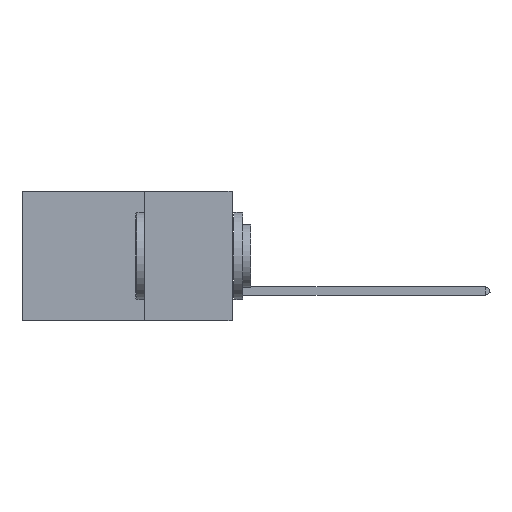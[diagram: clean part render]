
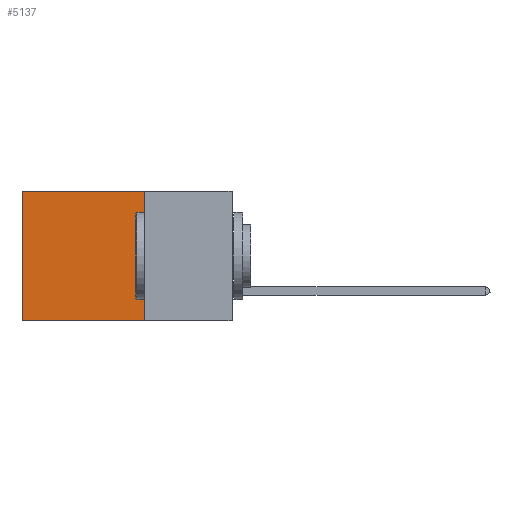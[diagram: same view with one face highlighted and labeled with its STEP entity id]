
A CAD part, left-side view. The second image highlights one B-rep face of the part: STEP entity #5137.
In plain terms, the highlighted planar face has unit normal (-1, 0, 0).
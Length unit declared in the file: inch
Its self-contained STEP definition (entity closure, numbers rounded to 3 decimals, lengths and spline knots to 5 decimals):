
#552 = LINE ( 'NONE', #20844, #25402 ) ;
#698 = CARTESIAN_POINT ( 'NONE',  ( 0.2875, 0.25, -0.37 ) ) ;
#1179 = DIRECTION ( 'NONE',  ( 0., 1., 0. ) ) ;
#1257 = LINE ( 'NONE', #7891, #14484 ) ;
#1474 = ORIENTED_EDGE ( 'NONE', *, *, #8886, .F. ) ;
#1738 = ORIENTED_EDGE ( 'NONE', *, *, #21145, .T. ) ;
#3791 = DIRECTION ( 'NONE',  ( 0., 0., -1. ) ) ;
#5137 = ADVANCED_FACE ( 'NONE', ( #21588 ), #13973, .F. ) ;
#6836 = EDGE_CURVE ( 'NONE', #13705, #20027, #1257, .T. ) ;
#7587 = CARTESIAN_POINT ( 'NONE',  ( 0.2875, 0.6, 0. ) ) ;
#7891 = CARTESIAN_POINT ( 'NONE',  ( 0.2875, 0.25, 0. ) ) ;
#8006 = CARTESIAN_POINT ( 'NONE',  ( 0.2875, 0.6, -0.37 ) ) ;
#8116 = VERTEX_POINT ( 'NONE', #698 ) ;
#8886 = EDGE_CURVE ( 'NONE', #8116, #20787, #552, .T. ) ;
#9477 = VECTOR ( 'NONE', #13708, 39.37008 ) ;
#11880 = DIRECTION ( 'NONE',  ( 0., 1., 0. ) ) ;
#13496 = CARTESIAN_POINT ( 'NONE',  ( 0.2875, 0.25, 0. ) ) ;
#13705 = VERTEX_POINT ( 'NONE', #17081 ) ;
#13708 = DIRECTION ( 'NONE',  ( 0., 0., -1. ) ) ;
#13969 = AXIS2_PLACEMENT_3D ( 'NONE', #22294, #14064, #3791 ) ;
#13973 = PLANE ( 'NONE',  #13969 ) ;
#14064 = DIRECTION ( 'NONE',  ( 1., 0., 0. ) ) ;
#14484 = VECTOR ( 'NONE', #11880, 39.37008 ) ;
#14541 = CARTESIAN_POINT ( 'NONE',  ( 0.2875, 0.6, 0. ) ) ;
#16172 = EDGE_CURVE ( 'NONE', #13705, #8116, #24617, .T. ) ;
#17081 = CARTESIAN_POINT ( 'NONE',  ( 0.2875, 0.25, 0. ) ) ;
#17193 = VECTOR ( 'NONE', #19395, 39.37008 ) ;
#19395 = DIRECTION ( 'NONE',  ( 0., 0., -1. ) ) ;
#19877 = EDGE_LOOP ( 'NONE', ( #1738, #1474, #21961, #25590 ) ) ;
#20027 = VERTEX_POINT ( 'NONE', #14541 ) ;
#20787 = VERTEX_POINT ( 'NONE', #8006 ) ;
#20844 = CARTESIAN_POINT ( 'NONE',  ( 0.2875, 0.25, -0.37 ) ) ;
#21145 = EDGE_CURVE ( 'NONE', #20027, #20787, #24647, .T. ) ;
#21588 = FACE_OUTER_BOUND ( 'NONE', #19877, .T. ) ;
#21961 = ORIENTED_EDGE ( 'NONE', *, *, #16172, .F. ) ;
#22294 = CARTESIAN_POINT ( 'NONE',  ( 0.2875, 0.25, 0. ) ) ;
#24617 = LINE ( 'NONE', #13496, #17193 ) ;
#24647 = LINE ( 'NONE', #7587, #9477 ) ;
#25402 = VECTOR ( 'NONE', #1179, 39.37008 ) ;
#25590 = ORIENTED_EDGE ( 'NONE', *, *, #6836, .T. ) ;
